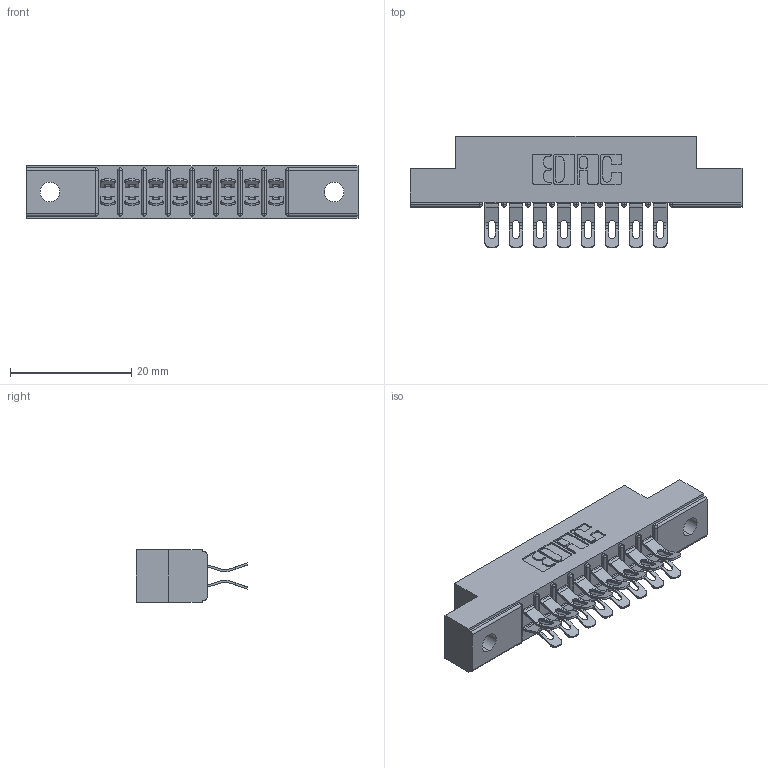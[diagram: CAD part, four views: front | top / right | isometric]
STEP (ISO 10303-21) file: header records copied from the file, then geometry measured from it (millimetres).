
FILE_DESCRIPTION (( 'STEP AP203' ), '1' );
FILE_NAME ('355-016-555-502.STEP', '2019-09-11T02:12:25', ( '' ), ( '' ), 'SwSTEP 2.0', 'SolidWorks 2016', '' );
FILE_SCHEMA (( 'CONFIG_CONTROL_DESIGN' ));
Length unit declared in the file: inch
Products named in the file (3): 355-016-555-502; 305 Part_.128 Dia; 305-290-001_555
Assembly tree (17 placements, depth 2):
  355-016-555-502
    305 Part_.128 Dia
    305-290-001_555  x16
Bounding box: 54.71 x 18.41 x 8.71 mm (x, y, z)
Volume: 3344.4 mm3; surface area: 5784.2 mm2
Topology: 17 solids, 17 shells, 1172 faces, 3476 edges, 2272 vertices
Faces by surface type: plane 580, cylinder 560, sphere 32
Entity records: 13427 total; most frequent: CARTESIAN_POINT 2240, ORIENTED_EDGE 2208, DIRECTION 2188, EDGE_CURVE 1104, VECTOR 836, LINE 836, VERTEX_POINT 712, AXIS2_PLACEMENT_3D 676
